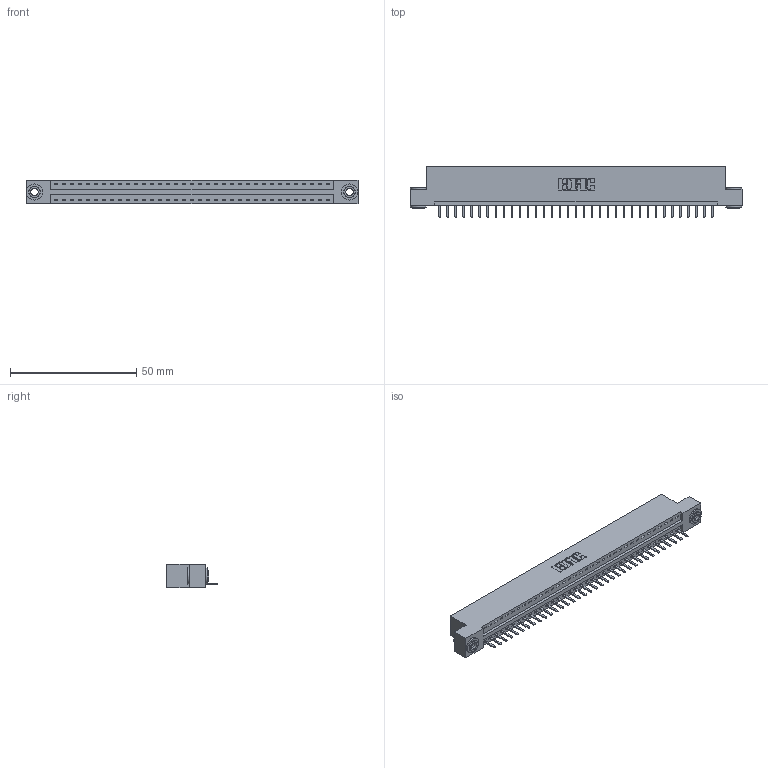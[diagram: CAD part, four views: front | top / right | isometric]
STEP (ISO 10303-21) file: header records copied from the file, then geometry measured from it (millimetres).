
FILE_DESCRIPTION (( 'STEP AP203' ), '1' );
FILE_NAME ('346-035-520-103.STEP', '2022-05-06T22:28:31', ( '' ), ( '' ), 'SwSTEP 2.0', 'SolidWorks 2020', '' );
FILE_SCHEMA (( 'CONFIG_CONTROL_DESIGN' ));
Length unit declared in the file: inch
Products named in the file (4): 346 Part_Flush Mounting Lugs - 0.156 Dia-TH; 345-250-002_345-250-002-102; 345-292-001_345-293-120; 346-035-520-103
Assembly tree (38 placements, depth 2):
  346-035-520-103
    346 Part_Flush Mounting Lugs - 0.156 Dia-TH
    345-292-001_345-293-120  x35
    345-250-002_345-250-002-102  x2
Bounding box: 131.7 x 20.02 x 9.4 mm (x, y, z)
Volume: 12458.9 mm3; surface area: 15411.9 mm2
Topology: 38 solids, 38 shells, 2344 faces, 6881 edges, 4490 vertices
Faces by surface type: plane 1570, cylinder 766, cone 8
Entity records: 23844 total; most frequent: CARTESIAN_POINT 4082, ORIENTED_EDGE 4030, DIRECTION 3627, EDGE_CURVE 2015, VECTOR 1715, LINE 1715, VERTEX_POINT 1338, AXIS2_PLACEMENT_3D 956
